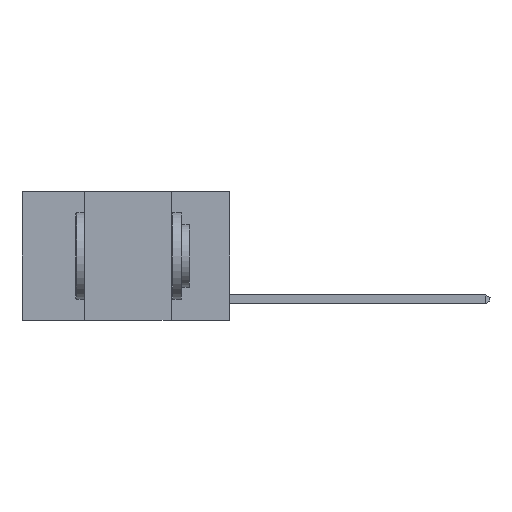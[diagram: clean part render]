
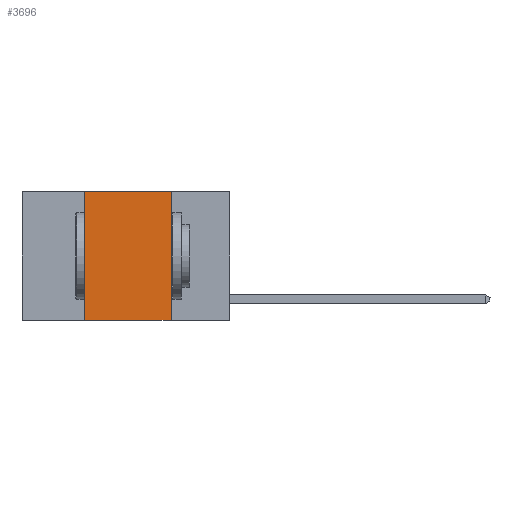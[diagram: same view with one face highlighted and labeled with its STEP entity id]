
A CAD part, left-side view. The second image highlights one B-rep face of the part: STEP entity #3696.
In plain terms, the highlighted planar face has unit normal (-1, 0, 0).
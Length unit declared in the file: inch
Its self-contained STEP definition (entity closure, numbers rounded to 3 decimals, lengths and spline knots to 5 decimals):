
#372 = DIRECTION ( 'NONE',  ( 0., -1., 0. ) ) ;
#1810 = FACE_OUTER_BOUND ( 'NONE', #19828, .T. ) ;
#2612 = AXIS2_PLACEMENT_3D ( 'NONE', #9290, #12940, #18724 ) ;
#2813 = LINE ( 'NONE', #22856, #4266 ) ;
#3549 = CARTESIAN_POINT ( 'NONE',  ( 0., 0.17, 0. ) ) ;
#3679 = CARTESIAN_POINT ( 'NONE',  ( 0., 0.42, 0. ) ) ;
#3696 = ADVANCED_FACE ( 'NONE', ( #1810 ), #14786, .F. ) ;
#4037 = VECTOR ( 'NONE', #20008, 39.37008 ) ;
#4266 = VECTOR ( 'NONE', #372, 39.37008 ) ;
#4552 = CARTESIAN_POINT ( 'NONE',  ( 0., 0.42, -0.37 ) ) ;
#5150 = LINE ( 'NONE', #8808, #22123 ) ;
#5772 = ORIENTED_EDGE ( 'NONE', *, *, #6562, .T. ) ;
#6562 = EDGE_CURVE ( 'NONE', #8239, #12813, #2813, .T. ) ;
#7766 = VERTEX_POINT ( 'NONE', #3549 ) ;
#8239 = VERTEX_POINT ( 'NONE', #4552 ) ;
#8808 = CARTESIAN_POINT ( 'NONE',  ( 0., 0.17, 0. ) ) ;
#9290 = CARTESIAN_POINT ( 'NONE',  ( 0., 0.6, 0. ) ) ;
#10760 = DIRECTION ( 'NONE',  ( 0., 0., -1. ) ) ;
#12504 = LINE ( 'NONE', #18164, #4037 ) ;
#12731 = EDGE_CURVE ( 'NONE', #7766, #12813, #5150, .T. ) ;
#12813 = VERTEX_POINT ( 'NONE', #17704 ) ;
#12940 = DIRECTION ( 'NONE',  ( 1., 0., 0. ) ) ;
#13537 = ORIENTED_EDGE ( 'NONE', *, *, #14904, .F. ) ;
#14052 = EDGE_CURVE ( 'NONE', #16158, #7766, #12504, .T. ) ;
#14786 = PLANE ( 'NONE',  #2612 ) ;
#14904 = EDGE_CURVE ( 'NONE', #8239, #16158, #23612, .T. ) ;
#16158 = VERTEX_POINT ( 'NONE', #3679 ) ;
#16297 = DIRECTION ( 'NONE',  ( 0., 0., 1. ) ) ;
#16643 = ORIENTED_EDGE ( 'NONE', *, *, #12731, .F. ) ;
#17704 = CARTESIAN_POINT ( 'NONE',  ( 0., 0.17, -0.37 ) ) ;
#18164 = CARTESIAN_POINT ( 'NONE',  ( 0., 0.6, 0. ) ) ;
#18659 = VECTOR ( 'NONE', #16297, 39.37008 ) ;
#18724 = DIRECTION ( 'NONE',  ( 0., 0., -1. ) ) ;
#18829 = ORIENTED_EDGE ( 'NONE', *, *, #14052, .F. ) ;
#19327 = CARTESIAN_POINT ( 'NONE',  ( 0., 0.42, 0. ) ) ;
#19828 = EDGE_LOOP ( 'NONE', ( #16643, #18829, #13537, #5772 ) ) ;
#20008 = DIRECTION ( 'NONE',  ( 0., -1., 0. ) ) ;
#22123 = VECTOR ( 'NONE', #10760, 39.37008 ) ;
#22856 = CARTESIAN_POINT ( 'NONE',  ( 0., 0.6, -0.37 ) ) ;
#23612 = LINE ( 'NONE', #19327, #18659 ) ;
